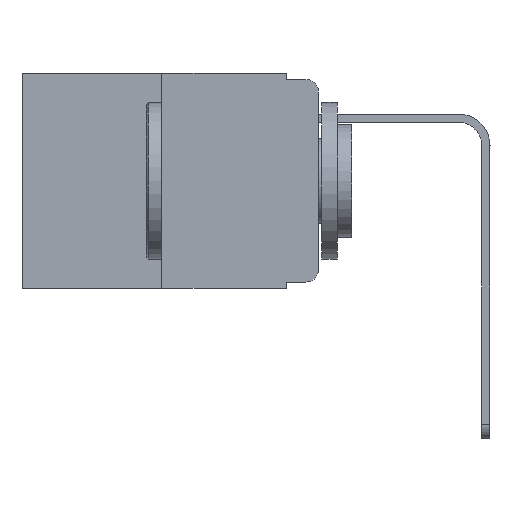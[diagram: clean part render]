
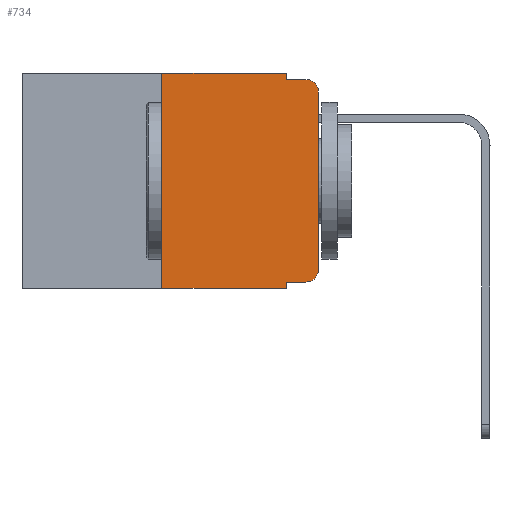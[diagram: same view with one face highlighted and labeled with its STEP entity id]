
A CAD part, left-side view. The second image highlights one B-rep face of the part: STEP entity #734.
In plain terms, the highlighted planar face has unit normal (-1, 0, 0).
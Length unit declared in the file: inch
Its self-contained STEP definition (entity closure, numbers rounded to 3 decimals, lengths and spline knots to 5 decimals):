
#110 = AXIS2_PLACEMENT_3D ( 'NONE', #11794, #8621, #219 ) ;
#219 = DIRECTION ( 'NONE',  ( 0., 0., -1. ) ) ;
#594 = DIRECTION ( 'NONE',  ( 0., 0., -1. ) ) ;
#644 = LINE ( 'NONE', #9962, #8736 ) ;
#734 = ADVANCED_FACE ( 'NONE', ( #4779 ), #6412, .F. ) ;
#1110 = DIRECTION ( 'NONE',  ( 1., 0., 0. ) ) ;
#1224 = EDGE_CURVE ( 'NONE', #11470, #13644, #9921, .T. ) ;
#1617 = CARTESIAN_POINT ( 'NONE',  ( 0., 0., -0.313 ) ) ;
#1636 = VERTEX_POINT ( 'NONE', #7268 ) ;
#1832 = ORIENTED_EDGE ( 'NONE', *, *, #1224, .T. ) ;
#2123 = CARTESIAN_POINT ( 'NONE',  ( 0., 0.473, 0. ) ) ;
#2325 = ORIENTED_EDGE ( 'NONE', *, *, #5861, .F. ) ;
#2603 = CARTESIAN_POINT ( 'NONE',  ( 0., 0.051, 0. ) ) ;
#2648 = VERTEX_POINT ( 'NONE', #13009 ) ;
#2748 = DIRECTION ( 'NONE',  ( 0., 0., -1. ) ) ;
#2789 = VERTEX_POINT ( 'NONE', #8872 ) ;
#2985 = VECTOR ( 'NONE', #5094, 39.37008 ) ;
#3094 = LINE ( 'NONE', #8040, #5581 ) ;
#3178 = VERTEX_POINT ( 'NONE', #2603 ) ;
#3553 = CARTESIAN_POINT ( 'NONE',  ( 0., 0.473, 0. ) ) ;
#3583 = DIRECTION ( 'NONE',  ( 0., 0., 1. ) ) ;
#3721 = CARTESIAN_POINT ( 'NONE',  ( 0., 0.25, -0.343 ) ) ;
#3823 = ORIENTED_EDGE ( 'NONE', *, *, #11918, .T. ) ;
#3999 = LINE ( 'NONE', #5878, #6482 ) ;
#4129 = EDGE_CURVE ( 'NONE', #13644, #2789, #8335, .T. ) ;
#4233 = EDGE_CURVE ( 'NONE', #8677, #3178, #9338, .T. ) ;
#4344 = VERTEX_POINT ( 'NONE', #10029 ) ;
#4779 = FACE_OUTER_BOUND ( 'NONE', #7713, .T. ) ;
#5048 = CARTESIAN_POINT ( 'NONE',  ( 0., 0.02, -0.333 ) ) ;
#5094 = DIRECTION ( 'NONE',  ( 0., -1., 0. ) ) ;
#5161 = ORIENTED_EDGE ( 'NONE', *, *, #6705, .T. ) ;
#5220 = VECTOR ( 'NONE', #10660, 39.37008 ) ;
#5443 = ORIENTED_EDGE ( 'NONE', *, *, #12313, .F. ) ;
#5581 = VECTOR ( 'NONE', #8738, 39.37008 ) ;
#5769 = CARTESIAN_POINT ( 'NONE',  ( 0., 0.051, -0.333 ) ) ;
#5861 = EDGE_CURVE ( 'NONE', #7906, #2648, #3999, .T. ) ;
#5878 = CARTESIAN_POINT ( 'NONE',  ( 0., 0.051, 0. ) ) ;
#5891 = VECTOR ( 'NONE', #2748, 39.37008 ) ;
#5940 = CARTESIAN_POINT ( 'NONE',  ( 0., 0.051, 0. ) ) ;
#6196 = LINE ( 'NONE', #5940, #5891 ) ;
#6247 = CARTESIAN_POINT ( 'NONE',  ( 0., 0.02, -0.03 ) ) ;
#6323 = CIRCLE ( 'NONE', #8338, 0.02 ) ;
#6364 = ORIENTED_EDGE ( 'NONE', *, *, #4129, .T. ) ;
#6412 = PLANE ( 'NONE',  #12756 ) ;
#6482 = VECTOR ( 'NONE', #594, 39.37008 ) ;
#6524 = VECTOR ( 'NONE', #10939, 39.37008 ) ;
#6705 = EDGE_CURVE ( 'NONE', #9192, #2648, #12403, .T. ) ;
#7268 = CARTESIAN_POINT ( 'NONE',  ( 0., 0.051, -0.01 ) ) ;
#7352 = DIRECTION ( 'NONE',  ( -1., 0., 0. ) ) ;
#7392 = EDGE_CURVE ( 'NONE', #2789, #4344, #6323, .T. ) ;
#7713 = EDGE_LOOP ( 'NONE', ( #6364, #13616, #5443, #12242, #10604, #11019, #5161, #2325, #3823, #1832 ) ) ;
#7906 = VERTEX_POINT ( 'NONE', #5769 ) ;
#8040 = CARTESIAN_POINT ( 'NONE',  ( 0., 0.051, -0.333 ) ) ;
#8335 = LINE ( 'NONE', #10802, #12470 ) ;
#8338 = AXIS2_PLACEMENT_3D ( 'NONE', #6247, #7352, #12669 ) ;
#8621 = DIRECTION ( 'NONE',  ( -1., 0., 0. ) ) ;
#8677 = VERTEX_POINT ( 'NONE', #10240 ) ;
#8736 = VECTOR ( 'NONE', #3583, 39.37008 ) ;
#8738 = DIRECTION ( 'NONE',  ( 0., -1., 0. ) ) ;
#8872 = CARTESIAN_POINT ( 'NONE',  ( 0., 0., -0.03 ) ) ;
#9192 = VERTEX_POINT ( 'NONE', #3721 ) ;
#9338 = LINE ( 'NONE', #3553, #6524 ) ;
#9612 = CARTESIAN_POINT ( 'NONE',  ( 0., 0.051, -0.01 ) ) ;
#9921 = CIRCLE ( 'NONE', #110, 0.02 ) ;
#9962 = CARTESIAN_POINT ( 'NONE',  ( 0., 0.25, 0. ) ) ;
#10029 = CARTESIAN_POINT ( 'NONE',  ( 0., 0.02, -0.01 ) ) ;
#10240 = CARTESIAN_POINT ( 'NONE',  ( 0., 0.25, 0. ) ) ;
#10581 = EDGE_CURVE ( 'NONE', #9192, #8677, #644, .T. ) ;
#10604 = ORIENTED_EDGE ( 'NONE', *, *, #4233, .F. ) ;
#10660 = DIRECTION ( 'NONE',  ( 0., -1., 0. ) ) ;
#10802 = CARTESIAN_POINT ( 'NONE',  ( 0., 0., 0. ) ) ;
#10939 = DIRECTION ( 'NONE',  ( 0., -1., 0. ) ) ;
#11019 = ORIENTED_EDGE ( 'NONE', *, *, #10581, .F. ) ;
#11470 = VERTEX_POINT ( 'NONE', #5048 ) ;
#11794 = CARTESIAN_POINT ( 'NONE',  ( 0., 0.02, -0.313 ) ) ;
#11816 = LINE ( 'NONE', #9612, #5220 ) ;
#11918 = EDGE_CURVE ( 'NONE', #7906, #11470, #3094, .T. ) ;
#12242 = ORIENTED_EDGE ( 'NONE', *, *, #12374, .F. ) ;
#12313 = EDGE_CURVE ( 'NONE', #1636, #4344, #11816, .T. ) ;
#12374 = EDGE_CURVE ( 'NONE', #3178, #1636, #6196, .T. ) ;
#12403 = LINE ( 'NONE', #13545, #2985 ) ;
#12470 = VECTOR ( 'NONE', #12930, 39.37008 ) ;
#12669 = DIRECTION ( 'NONE',  ( 0., 0., -1. ) ) ;
#12756 = AXIS2_PLACEMENT_3D ( 'NONE', #2123, #1110, #12787 ) ;
#12787 = DIRECTION ( 'NONE',  ( 0., 0., -1. ) ) ;
#12930 = DIRECTION ( 'NONE',  ( 0., 0., 1. ) ) ;
#13009 = CARTESIAN_POINT ( 'NONE',  ( 0., 0.051, -0.343 ) ) ;
#13545 = CARTESIAN_POINT ( 'NONE',  ( 0., 0.473, -0.343 ) ) ;
#13616 = ORIENTED_EDGE ( 'NONE', *, *, #7392, .T. ) ;
#13644 = VERTEX_POINT ( 'NONE', #1617 ) ;
